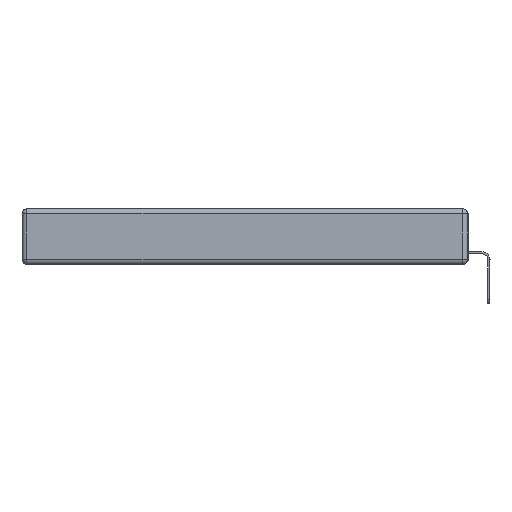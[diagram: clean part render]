
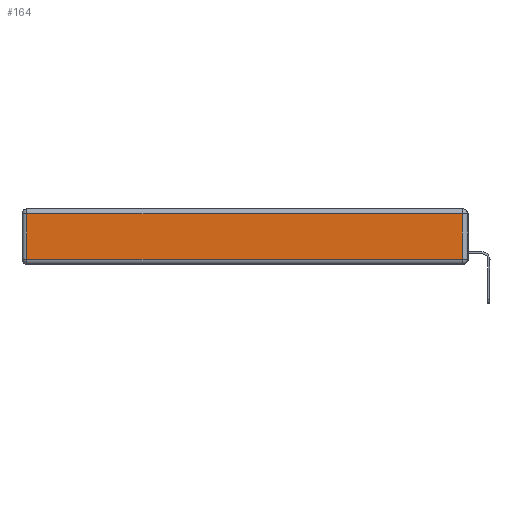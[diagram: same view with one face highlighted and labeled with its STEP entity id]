
A CAD part, left-side view. The second image highlights one B-rep face of the part: STEP entity #164.
In plain terms, the highlighted planar face has unit normal (-1, 0, 0).
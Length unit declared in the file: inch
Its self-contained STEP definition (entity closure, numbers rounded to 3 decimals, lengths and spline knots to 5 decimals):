
#164 = ADVANCED_FACE ( 'NONE', ( #16348 ), #20141, .T. ) ;
#519 = CARTESIAN_POINT ( 'NONE',  ( 0., 0., -0.343 ) ) ;
#651 = VECTOR ( 'NONE', #10935, 39.37008 ) ;
#843 = CARTESIAN_POINT ( 'NONE',  ( 0., 2.72, -0.03 ) ) ;
#1194 = AXIS2_PLACEMENT_3D ( 'NONE', #519, #14728, #20450 ) ;
#1392 = DIRECTION ( 'NONE',  ( 0., -1., 0. ) ) ;
#2177 = DIRECTION ( 'NONE',  ( 0., 0., 1. ) ) ;
#2460 = VERTEX_POINT ( 'NONE', #20711 ) ;
#2998 = ORIENTED_EDGE ( 'NONE', *, *, #20890, .T. ) ;
#4099 = CARTESIAN_POINT ( 'NONE',  ( 0., 0.03, -0.343 ) ) ;
#4316 = ORIENTED_EDGE ( 'NONE', *, *, #6114, .T. ) ;
#4471 = VERTEX_POINT ( 'NONE', #20797 ) ;
#5139 = CARTESIAN_POINT ( 'NONE',  ( 0., 0., -0.313 ) ) ;
#6114 = EDGE_CURVE ( 'NONE', #2460, #4471, #7008, .T. ) ;
#6829 = ORIENTED_EDGE ( 'NONE', *, *, #23160, .T. ) ;
#7008 = LINE ( 'NONE', #5139, #9810 ) ;
#7901 = LINE ( 'NONE', #20564, #15516 ) ;
#8487 = VECTOR ( 'NONE', #2177, 39.37008 ) ;
#8843 = ORIENTED_EDGE ( 'NONE', *, *, #10120, .T. ) ;
#9810 = VECTOR ( 'NONE', #1392, 39.37008 ) ;
#10120 = EDGE_CURVE ( 'NONE', #4471, #15403, #17513, .T. ) ;
#10935 = DIRECTION ( 'NONE',  ( 0., 1., 0. ) ) ;
#12746 = EDGE_LOOP ( 'NONE', ( #4316, #8843, #2998, #6829 ) ) ;
#14506 = VERTEX_POINT ( 'NONE', #843 ) ;
#14728 = DIRECTION ( 'NONE',  ( -1., 0., 0. ) ) ;
#15155 = DIRECTION ( 'NONE',  ( 0., 0., -1. ) ) ;
#15403 = VERTEX_POINT ( 'NONE', #21923 ) ;
#15516 = VECTOR ( 'NONE', #15155, 39.37008 ) ;
#16348 = FACE_OUTER_BOUND ( 'NONE', #12746, .T. ) ;
#17513 = LINE ( 'NONE', #4099, #8487 ) ;
#19632 = LINE ( 'NONE', #19938, #651 ) ;
#19938 = CARTESIAN_POINT ( 'NONE',  ( 0., 2.75, -0.03 ) ) ;
#20141 = PLANE ( 'NONE',  #1194 ) ;
#20450 = DIRECTION ( 'NONE',  ( 0., 0., 1. ) ) ;
#20564 = CARTESIAN_POINT ( 'NONE',  ( 0., 2.72, -0.343 ) ) ;
#20711 = CARTESIAN_POINT ( 'NONE',  ( 0., 2.72, -0.313 ) ) ;
#20797 = CARTESIAN_POINT ( 'NONE',  ( 0., 0.03, -0.313 ) ) ;
#20890 = EDGE_CURVE ( 'NONE', #15403, #14506, #19632, .T. ) ;
#21923 = CARTESIAN_POINT ( 'NONE',  ( 0., 0.03, -0.03 ) ) ;
#23160 = EDGE_CURVE ( 'NONE', #14506, #2460, #7901, .T. ) ;
